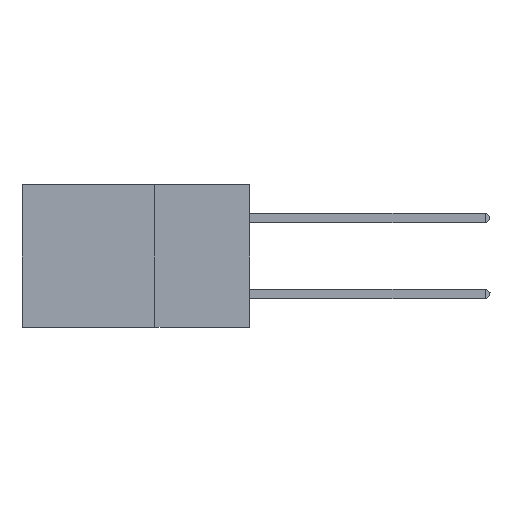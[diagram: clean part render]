
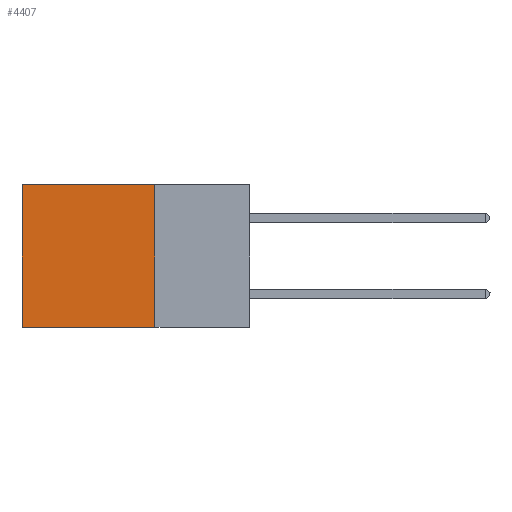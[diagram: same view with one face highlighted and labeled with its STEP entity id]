
A CAD part, left-side view. The second image highlights one B-rep face of the part: STEP entity #4407.
In plain terms, the highlighted planar face has unit normal (-1, 0, 0).
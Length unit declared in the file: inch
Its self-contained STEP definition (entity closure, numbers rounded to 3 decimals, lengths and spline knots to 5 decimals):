
#26 = DIRECTION ( 'NONE',  ( 0., 0., -1. ) ) ;
#141 = DIRECTION ( 'NONE',  ( 0., 0., -1. ) ) ;
#181 = VERTEX_POINT ( 'NONE', #12427 ) ;
#1546 = EDGE_CURVE ( 'NONE', #11039, #9051, #8853, .T. ) ;
#2391 = DIRECTION ( 'NONE',  ( 0., 1., 0. ) ) ;
#4407 = ADVANCED_FACE ( 'NONE', ( #8548 ), #11858, .F. ) ;
#5203 = DIRECTION ( 'NONE',  ( 1., 0., 0. ) ) ;
#5299 = CARTESIAN_POINT ( 'NONE',  ( 0.2875, 0.25, -0.375 ) ) ;
#6101 = LINE ( 'NONE', #7730, #13058 ) ;
#6578 = ORIENTED_EDGE ( 'NONE', *, *, #9377, .T. ) ;
#6716 = EDGE_CURVE ( 'NONE', #181, #8014, #9256, .T. ) ;
#7566 = CARTESIAN_POINT ( 'NONE',  ( 0.2875, 0.6, -0.375 ) ) ;
#7623 = CARTESIAN_POINT ( 'NONE',  ( 0.2875, 0.6, 0. ) ) ;
#7697 = VECTOR ( 'NONE', #8008, 39.37008 ) ;
#7730 = CARTESIAN_POINT ( 'NONE',  ( 0.2875, 0.25, -0.375 ) ) ;
#8008 = DIRECTION ( 'NONE',  ( 0., 1., 0. ) ) ;
#8014 = VERTEX_POINT ( 'NONE', #5299 ) ;
#8031 = ORIENTED_EDGE ( 'NONE', *, *, #6716, .F. ) ;
#8527 = LINE ( 'NONE', #9217, #7697 ) ;
#8548 = FACE_OUTER_BOUND ( 'NONE', #10439, .T. ) ;
#8626 = ORIENTED_EDGE ( 'NONE', *, *, #1546, .T. ) ;
#8796 = ORIENTED_EDGE ( 'NONE', *, *, #15949, .F. ) ;
#8853 = LINE ( 'NONE', #15851, #16639 ) ;
#9051 = VERTEX_POINT ( 'NONE', #7566 ) ;
#9109 = CARTESIAN_POINT ( 'NONE',  ( 0.2875, 0.25, -0.375 ) ) ;
#9217 = CARTESIAN_POINT ( 'NONE',  ( 0.2875, 0.25, 0. ) ) ;
#9256 = LINE ( 'NONE', #10395, #11529 ) ;
#9377 = EDGE_CURVE ( 'NONE', #181, #11039, #8527, .T. ) ;
#10395 = CARTESIAN_POINT ( 'NONE',  ( 0.2875, 0.25, -0.375 ) ) ;
#10439 = EDGE_LOOP ( 'NONE', ( #8626, #8796, #8031, #6578 ) ) ;
#11039 = VERTEX_POINT ( 'NONE', #7623 ) ;
#11529 = VECTOR ( 'NONE', #14777, 39.37008 ) ;
#11858 = PLANE ( 'NONE',  #11978 ) ;
#11978 = AXIS2_PLACEMENT_3D ( 'NONE', #9109, #5203, #26 ) ;
#12427 = CARTESIAN_POINT ( 'NONE',  ( 0.2875, 0.25, 0. ) ) ;
#13058 = VECTOR ( 'NONE', #2391, 39.37008 ) ;
#14777 = DIRECTION ( 'NONE',  ( 0., 0., -1. ) ) ;
#15851 = CARTESIAN_POINT ( 'NONE',  ( 0.2875, 0.6, -0.375 ) ) ;
#15949 = EDGE_CURVE ( 'NONE', #8014, #9051, #6101, .T. ) ;
#16639 = VECTOR ( 'NONE', #141, 39.37008 ) ;
